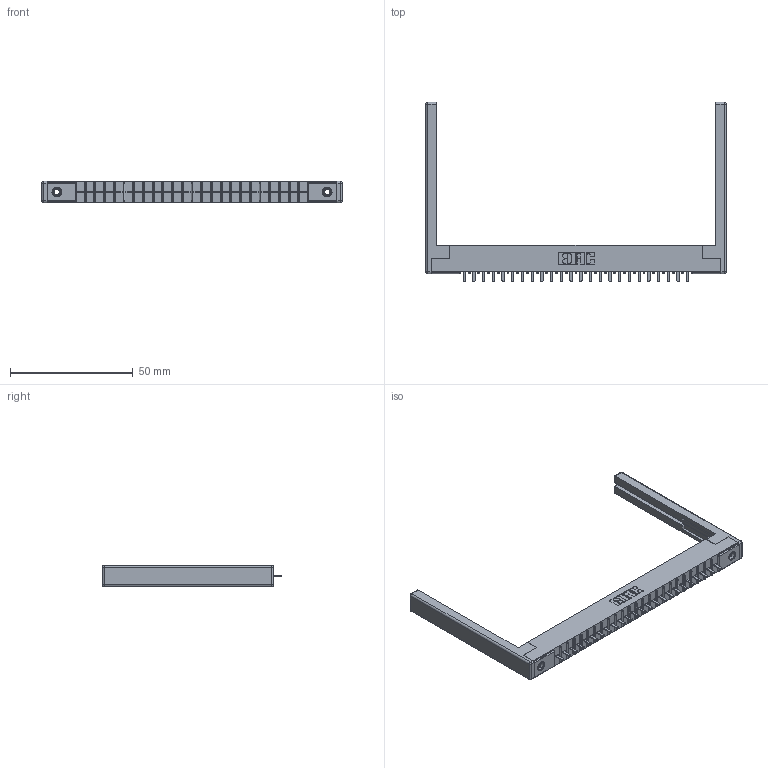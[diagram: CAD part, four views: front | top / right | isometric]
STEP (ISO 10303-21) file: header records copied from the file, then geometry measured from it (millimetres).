
FILE_DESCRIPTION (( 'STEP AP203' ), '1' );
FILE_NAME ('356-024-421-168.STEP', '2020-09-23T16:38:16', ( '' ), ( '' ), 'SwSTEP 2.0', 'SolidWorks 2020', '' );
FILE_SCHEMA (( 'CONFIG_CONTROL_DESIGN' ));
Length unit declared in the file: inch
Products named in the file (5): 306 Part_.156 Dia; 306-290-001_121; 345-250-001_345-250-001-102; 307-220-068; 356-024-421-168
Assembly tree (29 placements, depth 2):
  356-024-421-168
    306 Part_.156 Dia
    306-290-001_121  x24
    345-250-001_345-250-001-102  x2
    307-220-068  x2
Bounding box: 122.53 x 73.18 x 8.71 mm (x, y, z)
Volume: 12902.3 mm3; surface area: 16369.6 mm2
Topology: 29 solids, 29 shells, 1950 faces, 5434 edges, 3472 vertices
Faces by surface type: plane 1284, cylinder 546, sphere 104, cone 12, torus 4
Entity records: 27428 total; most frequent: CARTESIAN_POINT 4568, DIRECTION 4519, ORIENTED_EDGE 4518, EDGE_CURVE 2259, VECTOR 1753, LINE 1753, VERTEX_POINT 1432, AXIS2_PLACEMENT_3D 1383
